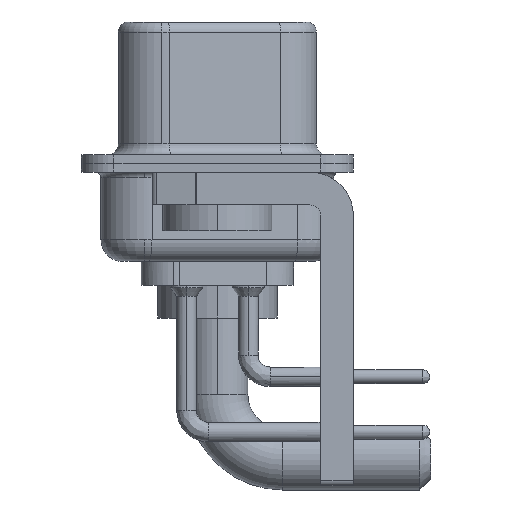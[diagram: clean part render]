
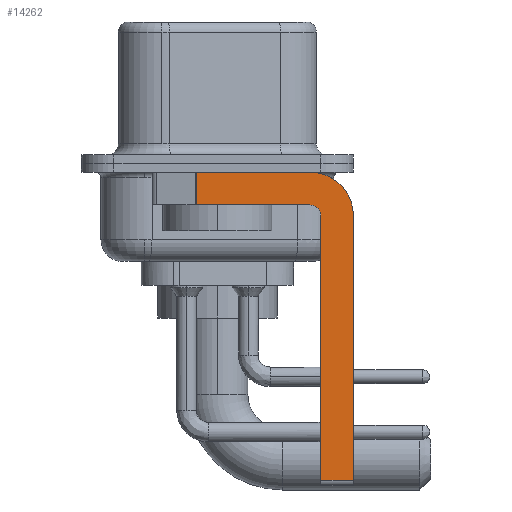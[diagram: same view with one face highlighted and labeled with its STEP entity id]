
A CAD part, left-side view. The second image highlights one B-rep face of the part: STEP entity #14262.
In plain terms, the highlighted planar face has unit normal (-1, 0, 0).
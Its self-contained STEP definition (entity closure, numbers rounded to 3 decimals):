
#109 = AXIS2_PLACEMENT_3D ( 'NONE', #15605, #7823, #9813 ) ;
#399 = LINE ( 'NONE', #18969, #16812 ) ;
#1125 = EDGE_CURVE ( 'NONE', #11288, #9839, #17968, .T. ) ;
#1176 = CARTESIAN_POINT ( 'NONE',  ( -2.9, 0.978, -1.9 ) ) ;
#1185 = DIRECTION ( 'NONE',  ( 0., 0., 1. ) ) ;
#2005 = EDGE_CURVE ( 'NONE', #19017, #10471, #11743, .T. ) ;
#2725 = CARTESIAN_POINT ( 'NONE',  ( -2.9, -4.75, -14.8 ) ) ;
#3168 = VECTOR ( 'NONE', #16640, 1000. ) ;
#3676 = CARTESIAN_POINT ( 'NONE',  ( -2.9, -6.25, -2.4 ) ) ;
#3864 = VECTOR ( 'NONE', #11310, 1000. ) ;
#4078 = ORIENTED_EDGE ( 'NONE', *, *, #1125, .T. ) ;
#4821 = EDGE_CURVE ( 'NONE', #14383, #8790, #4824, .T. ) ;
#4824 = LINE ( 'NONE', #12641, #3864 ) ;
#5299 = ORIENTED_EDGE ( 'NONE', *, *, #11027, .F. ) ;
#5531 = DIRECTION ( 'NONE',  ( -1., 0., 0. ) ) ;
#5769 = AXIS2_PLACEMENT_3D ( 'NONE', #10272, #5531, #8838 ) ;
#6080 = DIRECTION ( 'NONE',  ( 0., 0., -1. ) ) ;
#6198 = DIRECTION ( 'NONE',  ( 1., 0., 0. ) ) ;
#6638 = VECTOR ( 'NONE', #17323, 1000. ) ;
#6899 = ORIENTED_EDGE ( 'NONE', *, *, #4821, .F. ) ;
#7211 = CIRCLE ( 'NONE', #18991, 2. ) ;
#7334 = EDGE_CURVE ( 'NONE', #8790, #11788, #7211, .T. ) ;
#7654 = CARTESIAN_POINT ( 'NONE',  ( -2.9, -4.25, -0.4 ) ) ;
#7823 = DIRECTION ( 'NONE',  ( 1., 0., 0. ) ) ;
#8734 = CIRCLE ( 'NONE', #5769, 0.5 ) ;
#8790 = VERTEX_POINT ( 'NONE', #7654 ) ;
#8838 = DIRECTION ( 'NONE',  ( 0., 0., 1. ) ) ;
#9161 = CARTESIAN_POINT ( 'NONE',  ( -2.9, 0.978, -0.4 ) ) ;
#9354 = FACE_OUTER_BOUND ( 'NONE', #17987, .T. ) ;
#9480 = ORIENTED_EDGE ( 'NONE', *, *, #14437, .T. ) ;
#9813 = DIRECTION ( 'NONE',  ( 0., 0., -1. ) ) ;
#9839 = VERTEX_POINT ( 'NONE', #15520 ) ;
#10253 = CARTESIAN_POINT ( 'NONE',  ( -2.9, -4.75, -14.55 ) ) ;
#10272 = CARTESIAN_POINT ( 'NONE',  ( -2.9, -4.25, -2.4 ) ) ;
#10371 = VECTOR ( 'NONE', #11950, 1000. ) ;
#10471 = VERTEX_POINT ( 'NONE', #1176 ) ;
#10588 = VECTOR ( 'NONE', #1185, 1000. ) ;
#10645 = LINE ( 'NONE', #2725, #10588 ) ;
#11027 = EDGE_CURVE ( 'NONE', #11788, #9839, #14569, .T. ) ;
#11288 = VERTEX_POINT ( 'NONE', #10253 ) ;
#11310 = DIRECTION ( 'NONE',  ( 0., -1., 0. ) ) ;
#11743 = LINE ( 'NONE', #15119, #3168 ) ;
#11788 = VERTEX_POINT ( 'NONE', #18605 ) ;
#11950 = DIRECTION ( 'NONE',  ( 0., -1., 0. ) ) ;
#12641 = CARTESIAN_POINT ( 'NONE',  ( -2.9, 3., -0.4 ) ) ;
#12965 = ORIENTED_EDGE ( 'NONE', *, *, #2005, .F. ) ;
#13367 = EDGE_CURVE ( 'NONE', #11288, #13578, #10645, .T. ) ;
#13578 = VERTEX_POINT ( 'NONE', #15020 ) ;
#14017 = CARTESIAN_POINT ( 'NONE',  ( -2.9, -4.25, -1.9 ) ) ;
#14082 = PLANE ( 'NONE',  #109 ) ;
#14262 = ADVANCED_FACE ( 'NONE', ( #9354 ), #14082, .F. ) ;
#14383 = VERTEX_POINT ( 'NONE', #9161 ) ;
#14437 = EDGE_CURVE ( 'NONE', #14383, #10471, #399, .T. ) ;
#14569 = LINE ( 'NONE', #3676, #6638 ) ;
#14677 = ORIENTED_EDGE ( 'NONE', *, *, #18342, .F. ) ;
#14921 = CARTESIAN_POINT ( 'NONE',  ( -2.9, -4.25, -14.55 ) ) ;
#15020 = CARTESIAN_POINT ( 'NONE',  ( -2.9, -4.75, -2.4 ) ) ;
#15119 = CARTESIAN_POINT ( 'NONE',  ( -2.9, -4.25, -1.9 ) ) ;
#15436 = CARTESIAN_POINT ( 'NONE',  ( -2.9, -4.25, -2.4 ) ) ;
#15520 = CARTESIAN_POINT ( 'NONE',  ( -2.9, -6.25, -14.55 ) ) ;
#15605 = CARTESIAN_POINT ( 'NONE',  ( -2.9, -4.25, -2.4 ) ) ;
#16640 = DIRECTION ( 'NONE',  ( 0., 1., 0. ) ) ;
#16812 = VECTOR ( 'NONE', #19165, 1000. ) ;
#17129 = ORIENTED_EDGE ( 'NONE', *, *, #7334, .F. ) ;
#17323 = DIRECTION ( 'NONE',  ( 0., 0., -1. ) ) ;
#17968 = LINE ( 'NONE', #14921, #10371 ) ;
#17987 = EDGE_LOOP ( 'NONE', ( #6899, #9480, #12965, #14677, #19315, #4078, #5299, #17129 ) ) ;
#18342 = EDGE_CURVE ( 'NONE', #13578, #19017, #8734, .T. ) ;
#18605 = CARTESIAN_POINT ( 'NONE',  ( -2.9, -6.25, -2.4 ) ) ;
#18969 = CARTESIAN_POINT ( 'NONE',  ( -2.9, 0.978, -1.9 ) ) ;
#18991 = AXIS2_PLACEMENT_3D ( 'NONE', #15436, #6198, #6080 ) ;
#19017 = VERTEX_POINT ( 'NONE', #14017 ) ;
#19165 = DIRECTION ( 'NONE',  ( 0., 0., -1. ) ) ;
#19315 = ORIENTED_EDGE ( 'NONE', *, *, #13367, .F. ) ;
